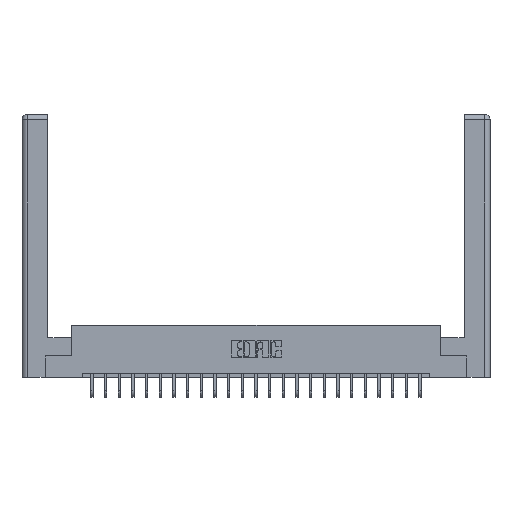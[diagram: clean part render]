
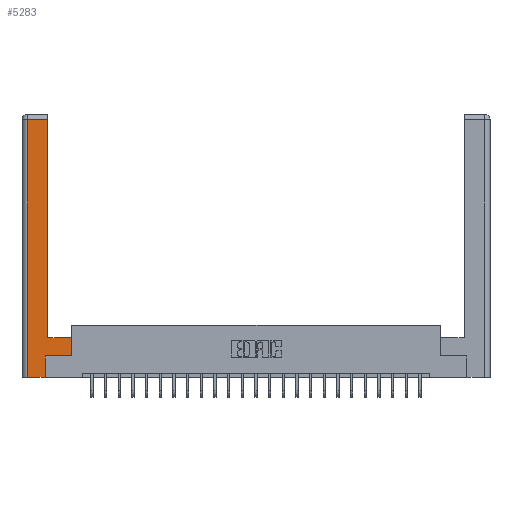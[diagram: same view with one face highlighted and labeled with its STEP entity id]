
A CAD part, top view. The second image highlights one B-rep face of the part: STEP entity #5283.
In plain terms, the highlighted planar face has unit normal (0, 0, 1).
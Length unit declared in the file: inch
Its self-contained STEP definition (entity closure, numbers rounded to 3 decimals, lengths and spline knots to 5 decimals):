
#466 = CARTESIAN_POINT ( 'NONE',  ( 0.0615, 0., 0. ) ) ;
#1973 = CARTESIAN_POINT ( 'NONE',  ( 0.565, 0.45, 0. ) ) ;
#2074 = VECTOR ( 'NONE', #6552, 39.37008 ) ;
#2099 = EDGE_CURVE ( 'NONE', #21009, #13500, #8340, .T. ) ;
#2195 = VERTEX_POINT ( 'NONE', #10377 ) ;
#2608 = EDGE_CURVE ( 'NONE', #13500, #16432, #11481, .T. ) ;
#3003 = VERTEX_POINT ( 'NONE', #18345 ) ;
#3026 = CARTESIAN_POINT ( 'NONE',  ( 0.265, 0.245, 0. ) ) ;
#3121 = DIRECTION ( 'NONE',  ( -1., 0., 0. ) ) ;
#3279 = VECTOR ( 'NONE', #4643, 39.37008 ) ;
#4185 = CARTESIAN_POINT ( 'NONE',  ( 0.265, 0., 0. ) ) ;
#4213 = CARTESIAN_POINT ( 'NONE',  ( 0.295, 3., 0. ) ) ;
#4625 = LINE ( 'NONE', #466, #14055 ) ;
#4637 = ORIENTED_EDGE ( 'NONE', *, *, #15255, .T. ) ;
#4643 = DIRECTION ( 'NONE',  ( 1., 0., 0. ) ) ;
#5283 = ADVANCED_FACE ( 'NONE', ( #23921 ), #17775, .F. ) ;
#5512 = LINE ( 'NONE', #4185, #2074 ) ;
#6117 = VECTOR ( 'NONE', #12108, 39.37008 ) ;
#6389 = ORIENTED_EDGE ( 'NONE', *, *, #20003, .T. ) ;
#6509 = DIRECTION ( 'NONE',  ( 0., 1., 0. ) ) ;
#6552 = DIRECTION ( 'NONE',  ( 1., 0., 0. ) ) ;
#6834 = EDGE_CURVE ( 'NONE', #2195, #14740, #20095, .T. ) ;
#7707 = VECTOR ( 'NONE', #10109, 39.37008 ) ;
#8008 = EDGE_LOOP ( 'NONE', ( #9153, #25644, #10777, #6389, #9804, #4637, #22572, #16725 ) ) ;
#8174 = CARTESIAN_POINT ( 'NONE',  ( 0.0615, 2.94, 0. ) ) ;
#8321 = EDGE_CURVE ( 'NONE', #9518, #21009, #21256, .T. ) ;
#8340 = LINE ( 'NONE', #4213, #7707 ) ;
#9153 = ORIENTED_EDGE ( 'NONE', *, *, #2099, .T. ) ;
#9347 = CARTESIAN_POINT ( 'NONE',  ( 0., 0., 0. ) ) ;
#9518 = VERTEX_POINT ( 'NONE', #1973 ) ;
#9804 = ORIENTED_EDGE ( 'NONE', *, *, #6834, .T. ) ;
#9991 = CARTESIAN_POINT ( 'NONE',  ( 0.0615, 2.94, 0. ) ) ;
#10109 = DIRECTION ( 'NONE',  ( 0., 1., 0. ) ) ;
#10175 = DIRECTION ( 'NONE',  ( 0., -1., 0. ) ) ;
#10377 = CARTESIAN_POINT ( 'NONE',  ( 0.265, 0., 0. ) ) ;
#10777 = ORIENTED_EDGE ( 'NONE', *, *, #13315, .T. ) ;
#11159 = LINE ( 'NONE', #15580, #25320 ) ;
#11377 = DIRECTION ( 'NONE',  ( 0., 0., -1. ) ) ;
#11481 = LINE ( 'NONE', #9991, #6117 ) ;
#11775 = VERTEX_POINT ( 'NONE', #20606 ) ;
#12108 = DIRECTION ( 'NONE',  ( -1., 0., 0. ) ) ;
#12412 = CARTESIAN_POINT ( 'NONE',  ( 0.265, 0.245, 0. ) ) ;
#12746 = CARTESIAN_POINT ( 'NONE',  ( 0.565, 0.245, 0. ) ) ;
#12964 = CARTESIAN_POINT ( 'NONE',  ( 0.295, 0.45, 0. ) ) ;
#13315 = EDGE_CURVE ( 'NONE', #16432, #3003, #4625, .T. ) ;
#13500 = VERTEX_POINT ( 'NONE', #22758 ) ;
#14055 = VECTOR ( 'NONE', #10175, 39.37008 ) ;
#14740 = VERTEX_POINT ( 'NONE', #3026 ) ;
#15255 = EDGE_CURVE ( 'NONE', #14740, #11775, #24978, .T. ) ;
#15580 = CARTESIAN_POINT ( 'NONE',  ( 0.565, 0.45, 0. ) ) ;
#16432 = VERTEX_POINT ( 'NONE', #8174 ) ;
#16725 = ORIENTED_EDGE ( 'NONE', *, *, #8321, .T. ) ;
#17227 = AXIS2_PLACEMENT_3D ( 'NONE', #9347, #11377, #25533 ) ;
#17693 = CARTESIAN_POINT ( 'NONE',  ( 0.295, 0.45, 0. ) ) ;
#17775 = PLANE ( 'NONE',  #17227 ) ;
#18345 = CARTESIAN_POINT ( 'NONE',  ( 0.0615, 0., 0. ) ) ;
#20003 = EDGE_CURVE ( 'NONE', #3003, #2195, #5512, .T. ) ;
#20095 = LINE ( 'NONE', #12412, #21648 ) ;
#20581 = EDGE_CURVE ( 'NONE', #11775, #9518, #11159, .T. ) ;
#20606 = CARTESIAN_POINT ( 'NONE',  ( 0.565, 0.245, 0. ) ) ;
#20627 = VECTOR ( 'NONE', #3121, 39.37008 ) ;
#21009 = VERTEX_POINT ( 'NONE', #12964 ) ;
#21256 = LINE ( 'NONE', #17693, #20627 ) ;
#21648 = VECTOR ( 'NONE', #6509, 39.37008 ) ;
#21661 = DIRECTION ( 'NONE',  ( 0., 1., 0. ) ) ;
#22572 = ORIENTED_EDGE ( 'NONE', *, *, #20581, .T. ) ;
#22758 = CARTESIAN_POINT ( 'NONE',  ( 0.295, 2.94, 0. ) ) ;
#23921 = FACE_OUTER_BOUND ( 'NONE', #8008, .T. ) ;
#24978 = LINE ( 'NONE', #12746, #3279 ) ;
#25320 = VECTOR ( 'NONE', #21661, 39.37008 ) ;
#25533 = DIRECTION ( 'NONE',  ( -1., 0., 0. ) ) ;
#25644 = ORIENTED_EDGE ( 'NONE', *, *, #2608, .T. ) ;
